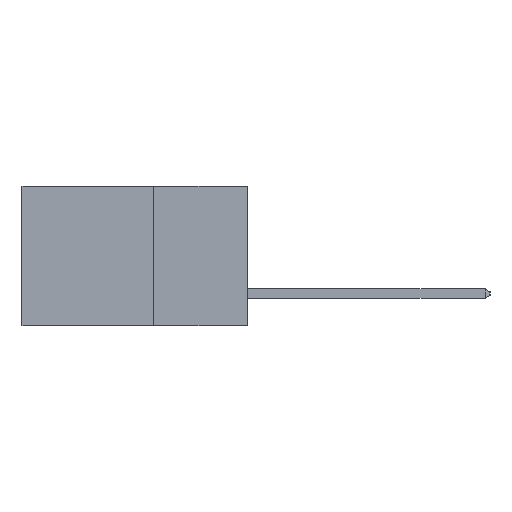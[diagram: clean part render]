
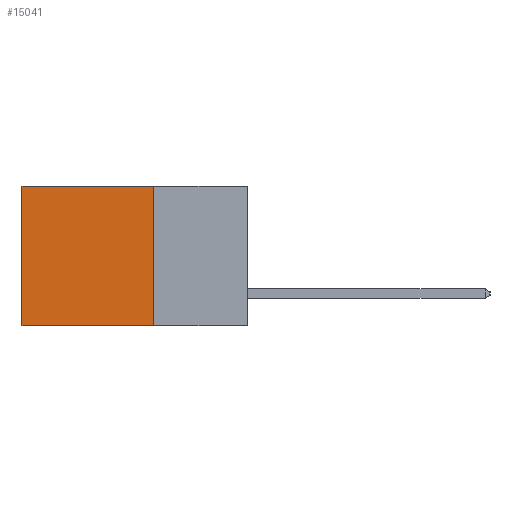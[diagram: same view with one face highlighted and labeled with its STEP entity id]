
A CAD part, left-side view. The second image highlights one B-rep face of the part: STEP entity #15041.
In plain terms, the highlighted planar face has unit normal (-1, 0, 0).
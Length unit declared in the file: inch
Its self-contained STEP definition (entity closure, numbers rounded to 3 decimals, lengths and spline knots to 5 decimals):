
#9 = LINE ( 'NONE', #4402, #23971 ) ;
#853 = CARTESIAN_POINT ( 'NONE',  ( 0.298, 0.25, 0. ) ) ;
#1152 = FACE_OUTER_BOUND ( 'NONE', #3825, .T. ) ;
#1617 = VERTEX_POINT ( 'NONE', #24879 ) ;
#1882 = VECTOR ( 'NONE', #7673, 39.37008 ) ;
#2048 = LINE ( 'NONE', #6124, #13642 ) ;
#3825 = EDGE_LOOP ( 'NONE', ( #13673, #5620, #29968, #28326 ) ) ;
#4402 = CARTESIAN_POINT ( 'NONE',  ( 0.298, 0.25, 0. ) ) ;
#5620 = ORIENTED_EDGE ( 'NONE', *, *, #16871, .F. ) ;
#6124 = CARTESIAN_POINT ( 'NONE',  ( 0.298, 0.25, 0. ) ) ;
#7150 = VERTEX_POINT ( 'NONE', #24276 ) ;
#7673 = DIRECTION ( 'NONE',  ( 0., 0., -1. ) ) ;
#10126 = EDGE_CURVE ( 'NONE', #10506, #24406, #9, .T. ) ;
#10506 = VERTEX_POINT ( 'NONE', #26563 ) ;
#11819 = EDGE_CURVE ( 'NONE', #10506, #7150, #2048, .T. ) ;
#13276 = LINE ( 'NONE', #16590, #18752 ) ;
#13642 = VECTOR ( 'NONE', #24795, 39.37008 ) ;
#13673 = ORIENTED_EDGE ( 'NONE', *, *, #14997, .T. ) ;
#14851 = DIRECTION ( 'NONE',  ( 0., 0., -1. ) ) ;
#14997 = EDGE_CURVE ( 'NONE', #7150, #1617, #20421, .T. ) ;
#15041 = ADVANCED_FACE ( 'NONE', ( #1152 ), #21777, .F. ) ;
#16017 = DIRECTION ( 'NONE',  ( 0., 0., -1. ) ) ;
#16590 = CARTESIAN_POINT ( 'NONE',  ( 0.298, 0.25, -0.37 ) ) ;
#16871 = EDGE_CURVE ( 'NONE', #24406, #1617, #13276, .T. ) ;
#18752 = VECTOR ( 'NONE', #25946, 39.37008 ) ;
#20421 = LINE ( 'NONE', #26236, #1882 ) ;
#21777 = PLANE ( 'NONE',  #22602 ) ;
#22602 = AXIS2_PLACEMENT_3D ( 'NONE', #853, #28765, #14851 ) ;
#23971 = VECTOR ( 'NONE', #16017, 39.37008 ) ;
#24276 = CARTESIAN_POINT ( 'NONE',  ( 0.298, 0.6, 0. ) ) ;
#24406 = VERTEX_POINT ( 'NONE', #28135 ) ;
#24795 = DIRECTION ( 'NONE',  ( 0., 1., 0. ) ) ;
#24879 = CARTESIAN_POINT ( 'NONE',  ( 0.298, 0.6, -0.37 ) ) ;
#25946 = DIRECTION ( 'NONE',  ( 0., 1., 0. ) ) ;
#26236 = CARTESIAN_POINT ( 'NONE',  ( 0.298, 0.6, 0. ) ) ;
#26563 = CARTESIAN_POINT ( 'NONE',  ( 0.298, 0.25, 0. ) ) ;
#28135 = CARTESIAN_POINT ( 'NONE',  ( 0.298, 0.25, -0.37 ) ) ;
#28326 = ORIENTED_EDGE ( 'NONE', *, *, #11819, .T. ) ;
#28765 = DIRECTION ( 'NONE',  ( 1., 0., 0. ) ) ;
#29968 = ORIENTED_EDGE ( 'NONE', *, *, #10126, .F. ) ;
